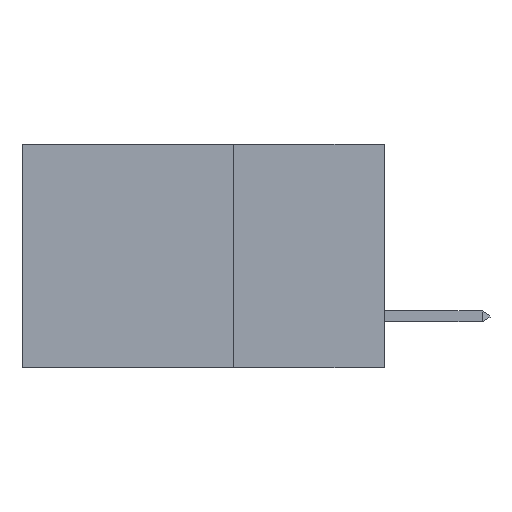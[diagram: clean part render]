
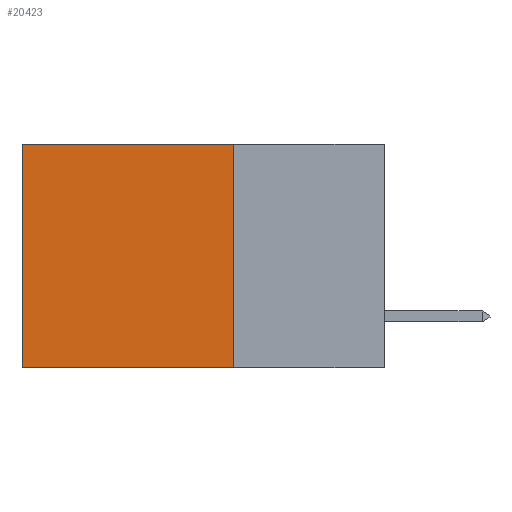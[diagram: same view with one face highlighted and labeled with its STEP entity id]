
A CAD part, left-side view. The second image highlights one B-rep face of the part: STEP entity #20423.
In plain terms, the highlighted planar face has unit normal (-1, 0, 0).
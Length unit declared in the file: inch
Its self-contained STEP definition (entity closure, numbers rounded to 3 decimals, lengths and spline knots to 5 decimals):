
#1320 = AXIS2_PLACEMENT_3D ( 'NONE', #14169, #3492, #15978 ) ;
#2497 = DIRECTION ( 'NONE',  ( 0., 0., -1. ) ) ;
#2925 = EDGE_CURVE ( 'NONE', #13334, #17181, #11047, .T. ) ;
#3492 = DIRECTION ( 'NONE',  ( 1., 0., 0. ) ) ;
#3555 = ORIENTED_EDGE ( 'NONE', *, *, #22606, .F. ) ;
#4659 = DIRECTION ( 'NONE',  ( 0., 0., -1. ) ) ;
#4829 = VERTEX_POINT ( 'NONE', #9967 ) ;
#6392 = VECTOR ( 'NONE', #2497, 39.37008 ) ;
#8153 = CARTESIAN_POINT ( 'NONE',  ( 0.2875, 0.25, -0.37 ) ) ;
#8297 = VERTEX_POINT ( 'NONE', #11982 ) ;
#8824 = PLANE ( 'NONE',  #1320 ) ;
#9091 = LINE ( 'NONE', #13304, #18326 ) ;
#9484 = ORIENTED_EDGE ( 'NONE', *, *, #22801, .T. ) ;
#9966 = CARTESIAN_POINT ( 'NONE',  ( 0.2875, 0.25, 0. ) ) ;
#9967 = CARTESIAN_POINT ( 'NONE',  ( 0.2875, 0.6, 0. ) ) ;
#10231 = VECTOR ( 'NONE', #20301, 39.37008 ) ;
#11047 = LINE ( 'NONE', #22407, #20471 ) ;
#11982 = CARTESIAN_POINT ( 'NONE',  ( 0.2875, 0.6, -0.37 ) ) ;
#13200 = CARTESIAN_POINT ( 'NONE',  ( 0.2875, 0.6, 0. ) ) ;
#13304 = CARTESIAN_POINT ( 'NONE',  ( 0.2875, 0.25, -0.37 ) ) ;
#13334 = VERTEX_POINT ( 'NONE', #9966 ) ;
#14169 = CARTESIAN_POINT ( 'NONE',  ( 0.2875, 0.25, 0. ) ) ;
#14388 = LINE ( 'NONE', #15017, #10231 ) ;
#14478 = EDGE_CURVE ( 'NONE', #4829, #8297, #15325, .T. ) ;
#15017 = CARTESIAN_POINT ( 'NONE',  ( 0.2875, 0.25, 0. ) ) ;
#15084 = DIRECTION ( 'NONE',  ( 0., 1., 0. ) ) ;
#15325 = LINE ( 'NONE', #13200, #6392 ) ;
#15978 = DIRECTION ( 'NONE',  ( 0., 0., -1. ) ) ;
#16052 = ORIENTED_EDGE ( 'NONE', *, *, #14478, .T. ) ;
#17181 = VERTEX_POINT ( 'NONE', #8153 ) ;
#17599 = EDGE_LOOP ( 'NONE', ( #16052, #3555, #19274, #9484 ) ) ;
#18326 = VECTOR ( 'NONE', #15084, 39.37008 ) ;
#19274 = ORIENTED_EDGE ( 'NONE', *, *, #2925, .F. ) ;
#20301 = DIRECTION ( 'NONE',  ( 0., 1., 0. ) ) ;
#20423 = ADVANCED_FACE ( 'NONE', ( #20843 ), #8824, .F. ) ;
#20471 = VECTOR ( 'NONE', #4659, 39.37008 ) ;
#20843 = FACE_OUTER_BOUND ( 'NONE', #17599, .T. ) ;
#22407 = CARTESIAN_POINT ( 'NONE',  ( 0.2875, 0.25, 0. ) ) ;
#22606 = EDGE_CURVE ( 'NONE', #17181, #8297, #9091, .T. ) ;
#22801 = EDGE_CURVE ( 'NONE', #13334, #4829, #14388, .T. ) ;
